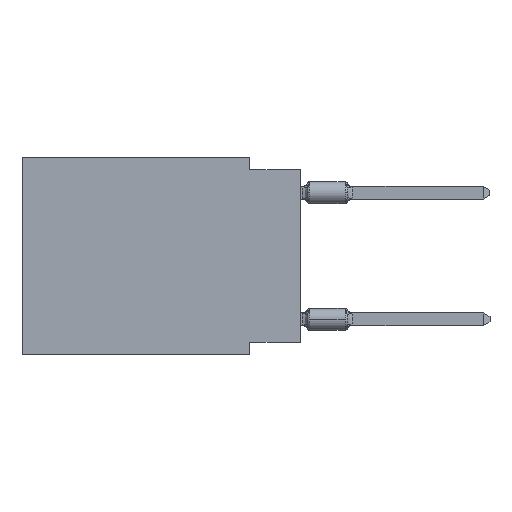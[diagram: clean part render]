
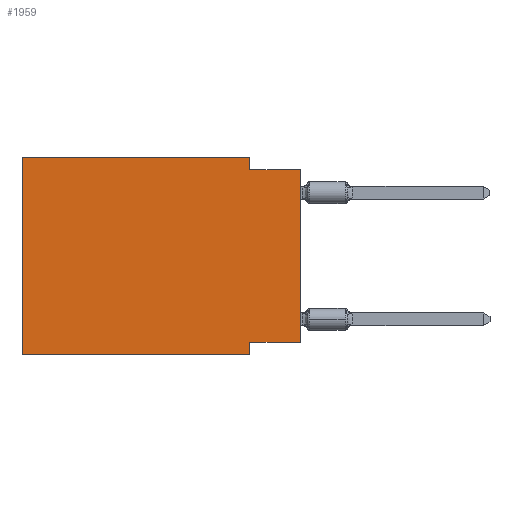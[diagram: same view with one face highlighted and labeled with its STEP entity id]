
A CAD part, left-side view. The second image highlights one B-rep face of the part: STEP entity #1959.
In plain terms, the highlighted planar face has unit normal (-1, 0, 0).
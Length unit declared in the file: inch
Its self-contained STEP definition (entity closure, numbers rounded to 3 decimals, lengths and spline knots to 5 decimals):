
#150 = VECTOR ( 'NONE', #18184, 39.37008 ) ;
#329 = LINE ( 'NONE', #7163, #150 ) ;
#341 = VERTEX_POINT ( 'NONE', #16689 ) ;
#884 = VERTEX_POINT ( 'NONE', #2779 ) ;
#887 = VERTEX_POINT ( 'NONE', #21052 ) ;
#1089 = CARTESIAN_POINT ( 'NONE',  ( 0., 0.55, 0. ) ) ;
#1237 = VECTOR ( 'NONE', #6503, 39.37008 ) ;
#1673 = DIRECTION ( 'NONE',  ( 0., -1., 0. ) ) ;
#1912 = LINE ( 'NONE', #8547, #7322 ) ;
#1959 = ADVANCED_FACE ( 'NONE', ( #5771 ), #15918, .F. ) ;
#2116 = VERTEX_POINT ( 'NONE', #16235 ) ;
#2203 = EDGE_CURVE ( 'NONE', #3048, #884, #329, .T. ) ;
#2779 = CARTESIAN_POINT ( 'NONE',  ( 0., 0.55, 0. ) ) ;
#3048 = VERTEX_POINT ( 'NONE', #11016 ) ;
#3460 = LINE ( 'NONE', #10058, #3693 ) ;
#3693 = VECTOR ( 'NONE', #11265, 39.37008 ) ;
#3986 = DIRECTION ( 'NONE',  ( 0., 0., -1. ) ) ;
#4046 = DIRECTION ( 'NONE',  ( 1., 0., 0. ) ) ;
#4291 = EDGE_CURVE ( 'NONE', #884, #18982, #10597, .T. ) ;
#4591 = EDGE_CURVE ( 'NONE', #341, #2116, #4644, .T. ) ;
#4644 = LINE ( 'NONE', #11448, #13634 ) ;
#4817 = ORIENTED_EDGE ( 'NONE', *, *, #13396, .F. ) ;
#5405 = VERTEX_POINT ( 'NONE', #19902 ) ;
#5771 = FACE_OUTER_BOUND ( 'NONE', #6457, .T. ) ;
#6034 = ORIENTED_EDGE ( 'NONE', *, *, #4591, .F. ) ;
#6457 = EDGE_LOOP ( 'NONE', ( #14786, #6034, #9829, #12114, #11686, #7918, #12869, #4817 ) ) ;
#6503 = DIRECTION ( 'NONE',  ( 0., 0., -1. ) ) ;
#7034 = CARTESIAN_POINT ( 'NONE',  ( 0., 0.55, 0. ) ) ;
#7163 = CARTESIAN_POINT ( 'NONE',  ( 0., 0.55, 0. ) ) ;
#7322 = VECTOR ( 'NONE', #3986, 39.37008 ) ;
#7707 = DIRECTION ( 'NONE',  ( 0., 0., -1. ) ) ;
#7918 = ORIENTED_EDGE ( 'NONE', *, *, #19427, .T. ) ;
#8547 = CARTESIAN_POINT ( 'NONE',  ( 0., 0.1, -0.39 ) ) ;
#8908 = EDGE_CURVE ( 'NONE', #5405, #2116, #17203, .T. ) ;
#9829 = ORIENTED_EDGE ( 'NONE', *, *, #18533, .F. ) ;
#10058 = CARTESIAN_POINT ( 'NONE',  ( 0., 0.55, -0.39 ) ) ;
#10597 = LINE ( 'NONE', #7034, #15421 ) ;
#10605 = DIRECTION ( 'NONE',  ( 0., 0., 1. ) ) ;
#11016 = CARTESIAN_POINT ( 'NONE',  ( 0., 0.55, -0.39 ) ) ;
#11265 = DIRECTION ( 'NONE',  ( 0., -1., 0. ) ) ;
#11387 = VECTOR ( 'NONE', #10605, 39.37008 ) ;
#11448 = CARTESIAN_POINT ( 'NONE',  ( 0., 0., -0.025 ) ) ;
#11571 = EDGE_CURVE ( 'NONE', #887, #13251, #1912, .T. ) ;
#11686 = ORIENTED_EDGE ( 'NONE', *, *, #2203, .F. ) ;
#11892 = DIRECTION ( 'NONE',  ( 0., -1., 0. ) ) ;
#12114 = ORIENTED_EDGE ( 'NONE', *, *, #4291, .F. ) ;
#12606 = DIRECTION ( 'NONE',  ( 0., 1., 0. ) ) ;
#12869 = ORIENTED_EDGE ( 'NONE', *, *, #11571, .F. ) ;
#13216 = CARTESIAN_POINT ( 'NONE',  ( 0., 0.1, 0. ) ) ;
#13251 = VERTEX_POINT ( 'NONE', #20172 ) ;
#13396 = EDGE_CURVE ( 'NONE', #5405, #887, #21026, .T. ) ;
#13420 = CARTESIAN_POINT ( 'NONE',  ( 0., 0.1, 0. ) ) ;
#13523 = CARTESIAN_POINT ( 'NONE',  ( 0., 0., 0. ) ) ;
#13534 = VECTOR ( 'NONE', #12606, 39.37008 ) ;
#13634 = VECTOR ( 'NONE', #1673, 39.37008 ) ;
#14323 = CARTESIAN_POINT ( 'NONE',  ( 0., 0., -0.365 ) ) ;
#14786 = ORIENTED_EDGE ( 'NONE', *, *, #8908, .T. ) ;
#15136 = LINE ( 'NONE', #13420, #1237 ) ;
#15421 = VECTOR ( 'NONE', #11892, 39.37008 ) ;
#15918 = PLANE ( 'NONE',  #18796 ) ;
#16235 = CARTESIAN_POINT ( 'NONE',  ( 0., 0., -0.025 ) ) ;
#16689 = CARTESIAN_POINT ( 'NONE',  ( 0., 0.1, -0.025 ) ) ;
#17203 = LINE ( 'NONE', #13523, #11387 ) ;
#18184 = DIRECTION ( 'NONE',  ( 0., 0., 1. ) ) ;
#18533 = EDGE_CURVE ( 'NONE', #18982, #341, #15136, .T. ) ;
#18796 = AXIS2_PLACEMENT_3D ( 'NONE', #1089, #4046, #7707 ) ;
#18982 = VERTEX_POINT ( 'NONE', #13216 ) ;
#19427 = EDGE_CURVE ( 'NONE', #3048, #13251, #3460, .T. ) ;
#19902 = CARTESIAN_POINT ( 'NONE',  ( 0., 0., -0.365 ) ) ;
#20172 = CARTESIAN_POINT ( 'NONE',  ( 0., 0.1, -0.39 ) ) ;
#21026 = LINE ( 'NONE', #14323, #13534 ) ;
#21052 = CARTESIAN_POINT ( 'NONE',  ( 0., 0.1, -0.365 ) ) ;
